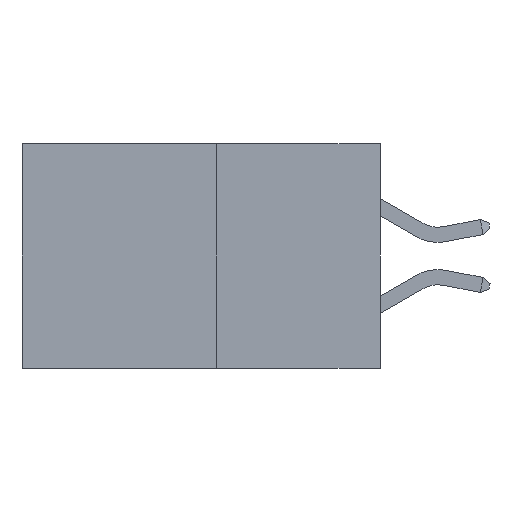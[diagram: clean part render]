
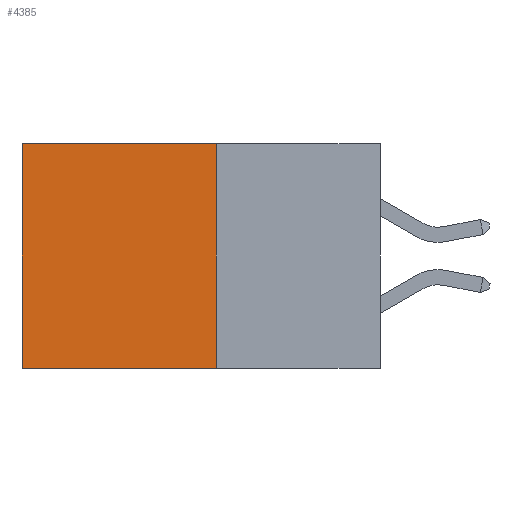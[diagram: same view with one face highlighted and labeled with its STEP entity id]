
A CAD part, left-side view. The second image highlights one B-rep face of the part: STEP entity #4385.
In plain terms, the highlighted planar face has unit normal (-1, 0, 0).
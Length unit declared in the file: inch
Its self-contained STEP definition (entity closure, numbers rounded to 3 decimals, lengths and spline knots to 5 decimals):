
#15 = CARTESIAN_POINT ( 'NONE',  ( 0.277, 0.27, -0.37 ) ) ;
#18 = VECTOR ( 'NONE', #5529, 39.37008 ) ;
#135 = ORIENTED_EDGE ( 'NONE', *, *, #5415, .T. ) ;
#152 = CARTESIAN_POINT ( 'NONE',  ( 0.277, 0.27, -0.37 ) ) ;
#438 = DIRECTION ( 'NONE',  ( 0., 1., 0. ) ) ;
#734 = EDGE_CURVE ( 'NONE', #8296, #1109, #6866, .T. ) ;
#751 = FACE_OUTER_BOUND ( 'NONE', #9293, .T. ) ;
#1109 = VERTEX_POINT ( 'NONE', #15 ) ;
#2133 = ORIENTED_EDGE ( 'NONE', *, *, #734, .F. ) ;
#2354 = ORIENTED_EDGE ( 'NONE', *, *, #6447, .F. ) ;
#2619 = EDGE_CURVE ( 'NONE', #8296, #10579, #10025, .T. ) ;
#4385 = ADVANCED_FACE ( 'NONE', ( #751 ), #10440, .F. ) ;
#5339 = VECTOR ( 'NONE', #8160, 39.37008 ) ;
#5415 = EDGE_CURVE ( 'NONE', #10579, #6091, #10625, .T. ) ;
#5514 = CARTESIAN_POINT ( 'NONE',  ( 0.277, 0.27, 0. ) ) ;
#5529 = DIRECTION ( 'NONE',  ( 0., 0., -1. ) ) ;
#6091 = VERTEX_POINT ( 'NONE', #7315 ) ;
#6447 = EDGE_CURVE ( 'NONE', #1109, #6091, #6455, .T. ) ;
#6455 = LINE ( 'NONE', #152, #10849 ) ;
#6866 = LINE ( 'NONE', #8815, #18 ) ;
#7315 = CARTESIAN_POINT ( 'NONE',  ( 0.277, 0.59, -0.37 ) ) ;
#8160 = DIRECTION ( 'NONE',  ( 0., 1., 0. ) ) ;
#8276 = ORIENTED_EDGE ( 'NONE', *, *, #2619, .T. ) ;
#8296 = VERTEX_POINT ( 'NONE', #5514 ) ;
#8815 = CARTESIAN_POINT ( 'NONE',  ( 0.277, 0.27, -0.37 ) ) ;
#9111 = CARTESIAN_POINT ( 'NONE',  ( 0.277, 0.59, 0. ) ) ;
#9293 = EDGE_LOOP ( 'NONE', ( #135, #2354, #2133, #8276 ) ) ;
#9360 = CARTESIAN_POINT ( 'NONE',  ( 0.277, 0.59, -0.37 ) ) ;
#9568 = DIRECTION ( 'NONE',  ( 0., 0., -1. ) ) ;
#10025 = LINE ( 'NONE', #11137, #5339 ) ;
#10135 = DIRECTION ( 'NONE',  ( 0., 0., -1. ) ) ;
#10356 = VECTOR ( 'NONE', #9568, 39.37008 ) ;
#10399 = DIRECTION ( 'NONE',  ( 1., 0., 0. ) ) ;
#10440 = PLANE ( 'NONE',  #11174 ) ;
#10507 = CARTESIAN_POINT ( 'NONE',  ( 0.277, 0.27, -0.37 ) ) ;
#10579 = VERTEX_POINT ( 'NONE', #9111 ) ;
#10625 = LINE ( 'NONE', #9360, #10356 ) ;
#10849 = VECTOR ( 'NONE', #438, 39.37008 ) ;
#11137 = CARTESIAN_POINT ( 'NONE',  ( 0.277, 0.27, 0. ) ) ;
#11174 = AXIS2_PLACEMENT_3D ( 'NONE', #10507, #10399, #10135 ) ;
